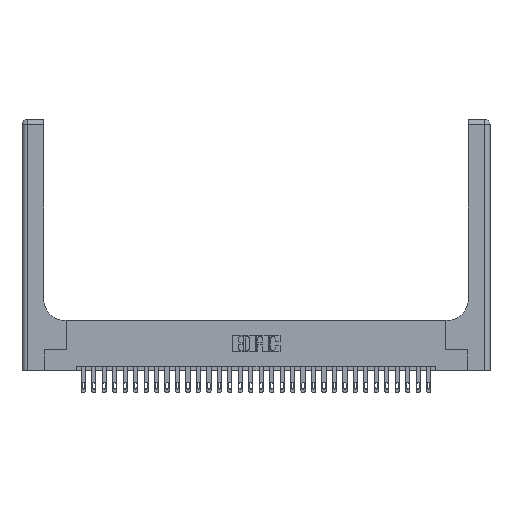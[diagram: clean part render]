
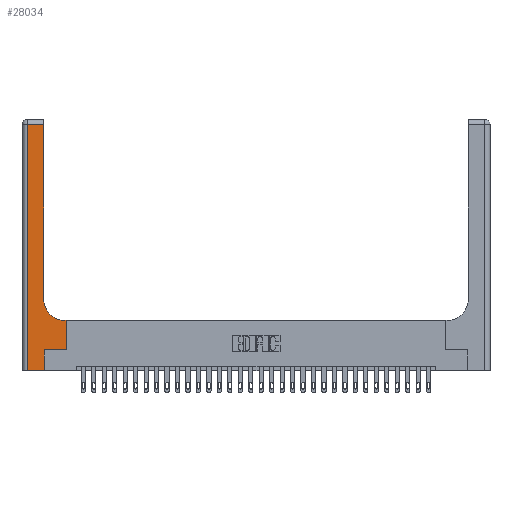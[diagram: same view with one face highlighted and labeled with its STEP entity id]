
A CAD part, top view. The second image highlights one B-rep face of the part: STEP entity #28034.
In plain terms, the highlighted planar face has unit normal (0, 0, 1).
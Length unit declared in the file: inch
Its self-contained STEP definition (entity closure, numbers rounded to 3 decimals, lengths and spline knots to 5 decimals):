
#81 = CARTESIAN_POINT ( 'NONE',  ( 0.26, 0.6, 0.37 ) ) ;
#669 = CARTESIAN_POINT ( 'NONE',  ( 0.26, 2.94, 0.37 ) ) ;
#1248 = DIRECTION ( 'NONE',  ( 0., -1., 0. ) ) ;
#1342 = LINE ( 'NONE', #20789, #16041 ) ;
#2142 = VERTEX_POINT ( 'NONE', #669 ) ;
#2311 = EDGE_CURVE ( 'NONE', #26471, #20106, #3148, .T. ) ;
#3148 = LINE ( 'NONE', #11883, #26781 ) ;
#3448 = EDGE_CURVE ( 'NONE', #19150, #2142, #10913, .T. ) ;
#3552 = CARTESIAN_POINT ( 'NONE',  ( 0.51, 0.6, 0.37 ) ) ;
#4372 = DIRECTION ( 'NONE',  ( 0., 0., -1. ) ) ;
#4749 = CIRCLE ( 'NONE', #14945, 0.25 ) ;
#5123 = EDGE_CURVE ( 'NONE', #25208, #19150, #4749, .T. ) ;
#5371 = EDGE_CURVE ( 'NONE', #20106, #25208, #24899, .T. ) ;
#5932 = DIRECTION ( 'NONE',  ( 1., 0., 0. ) ) ;
#6535 = VERTEX_POINT ( 'NONE', #18919 ) ;
#7599 = DIRECTION ( 'NONE',  ( 0., 1., 0. ) ) ;
#7852 = ORIENTED_EDGE ( 'NONE', *, *, #19117, .T. ) ;
#8119 = LINE ( 'NONE', #23890, #21577 ) ;
#8344 = VERTEX_POINT ( 'NONE', #24430 ) ;
#8440 = CARTESIAN_POINT ( 'NONE',  ( 0.528, 0.25, 0.37 ) ) ;
#8638 = EDGE_CURVE ( 'NONE', #2142, #24517, #1342, .T. ) ;
#8726 = CARTESIAN_POINT ( 'NONE',  ( 0., 3., 0.37 ) ) ;
#9991 = ORIENTED_EDGE ( 'NONE', *, *, #8638, .T. ) ;
#10357 = ORIENTED_EDGE ( 'NONE', *, *, #3448, .T. ) ;
#10913 = LINE ( 'NONE', #26828, #21421 ) ;
#11883 = CARTESIAN_POINT ( 'NONE',  ( 0.528, 0.25, 0.37 ) ) ;
#12154 = VERTEX_POINT ( 'NONE', #18530 ) ;
#12395 = ORIENTED_EDGE ( 'NONE', *, *, #5123, .T. ) ;
#12430 = DIRECTION ( 'NONE',  ( 1., 0., 0. ) ) ;
#14061 = DIRECTION ( 'NONE',  ( 0., 1., 0. ) ) ;
#14673 = CARTESIAN_POINT ( 'NONE',  ( 0.51, 0.85, 0.37 ) ) ;
#14806 = DIRECTION ( 'NONE',  ( 1., 0., 0. ) ) ;
#14924 = CARTESIAN_POINT ( 'NONE',  ( 0.06, 3., 0.37 ) ) ;
#14945 = AXIS2_PLACEMENT_3D ( 'NONE', #14673, #23886, #14806 ) ;
#15445 = FACE_OUTER_BOUND ( 'NONE', #27940, .T. ) ;
#15736 = PLANE ( 'NONE',  #22641 ) ;
#15820 = DIRECTION ( 'NONE',  ( -1., 0., 0. ) ) ;
#16041 = VECTOR ( 'NONE', #16516, 39.37008 ) ;
#16516 = DIRECTION ( 'NONE',  ( -1., 0., 0. ) ) ;
#16961 = LINE ( 'NONE', #21509, #24795 ) ;
#18280 = ORIENTED_EDGE ( 'NONE', *, *, #23962, .T. ) ;
#18362 = ORIENTED_EDGE ( 'NONE', *, *, #5371, .T. ) ;
#18530 = CARTESIAN_POINT ( 'NONE',  ( 0.265, 0., 0.37 ) ) ;
#18919 = CARTESIAN_POINT ( 'NONE',  ( 0.265, 0.25, 0.37 ) ) ;
#19117 = EDGE_CURVE ( 'NONE', #6535, #26471, #16961, .T. ) ;
#19150 = VERTEX_POINT ( 'NONE', #26587 ) ;
#20106 = VERTEX_POINT ( 'NONE', #24902 ) ;
#20170 = VECTOR ( 'NONE', #7599, 39.37008 ) ;
#20789 = CARTESIAN_POINT ( 'NONE',  ( 0., 2.94, 0.37 ) ) ;
#21296 = ORIENTED_EDGE ( 'NONE', *, *, #28748, .T. ) ;
#21421 = VECTOR ( 'NONE', #22027, 39.37008 ) ;
#21509 = CARTESIAN_POINT ( 'NONE',  ( 0.265, 0.25, 0.37 ) ) ;
#21565 = CARTESIAN_POINT ( 'NONE',  ( 0.06, 2.94, 0.37 ) ) ;
#21577 = VECTOR ( 'NONE', #5932, 39.37008 ) ;
#22027 = DIRECTION ( 'NONE',  ( 0., 1., 0. ) ) ;
#22186 = DIRECTION ( 'NONE',  ( -1., 0., 0. ) ) ;
#22641 = AXIS2_PLACEMENT_3D ( 'NONE', #8726, #4372, #22186 ) ;
#23747 = ORIENTED_EDGE ( 'NONE', *, *, #2311, .T. ) ;
#23886 = DIRECTION ( 'NONE',  ( 0., 0., -1. ) ) ;
#23890 = CARTESIAN_POINT ( 'NONE',  ( 0., 0., 0.37 ) ) ;
#23962 = EDGE_CURVE ( 'NONE', #12154, #6535, #27595, .T. ) ;
#24430 = CARTESIAN_POINT ( 'NONE',  ( 0.06, 0., 0.37 ) ) ;
#24472 = EDGE_CURVE ( 'NONE', #8344, #12154, #8119, .T. ) ;
#24514 = VECTOR ( 'NONE', #1248, 39.37008 ) ;
#24517 = VERTEX_POINT ( 'NONE', #21565 ) ;
#24795 = VECTOR ( 'NONE', #12430, 39.37008 ) ;
#24899 = LINE ( 'NONE', #81, #25114 ) ;
#24902 = CARTESIAN_POINT ( 'NONE',  ( 0.528, 0.6, 0.37 ) ) ;
#24994 = ORIENTED_EDGE ( 'NONE', *, *, #24472, .T. ) ;
#25114 = VECTOR ( 'NONE', #15820, 39.37008 ) ;
#25208 = VERTEX_POINT ( 'NONE', #3552 ) ;
#26033 = LINE ( 'NONE', #14924, #24514 ) ;
#26471 = VERTEX_POINT ( 'NONE', #8440 ) ;
#26587 = CARTESIAN_POINT ( 'NONE',  ( 0.26, 0.85, 0.37 ) ) ;
#26781 = VECTOR ( 'NONE', #14061, 39.37008 ) ;
#26828 = CARTESIAN_POINT ( 'NONE',  ( 0.26, 3., 0.37 ) ) ;
#27595 = LINE ( 'NONE', #27738, #20170 ) ;
#27738 = CARTESIAN_POINT ( 'NONE',  ( 0.265, 0., 0.37 ) ) ;
#27940 = EDGE_LOOP ( 'NONE', ( #10357, #9991, #21296, #24994, #18280, #7852, #23747, #18362, #12395 ) ) ;
#28034 = ADVANCED_FACE ( 'NONE', ( #15445 ), #15736, .F. ) ;
#28748 = EDGE_CURVE ( 'NONE', #24517, #8344, #26033, .T. ) ;
